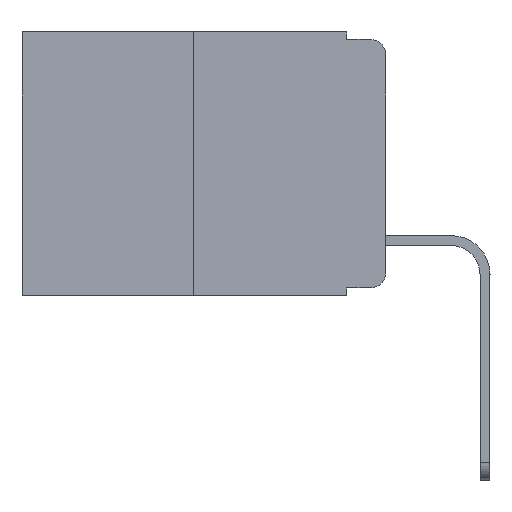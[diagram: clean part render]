
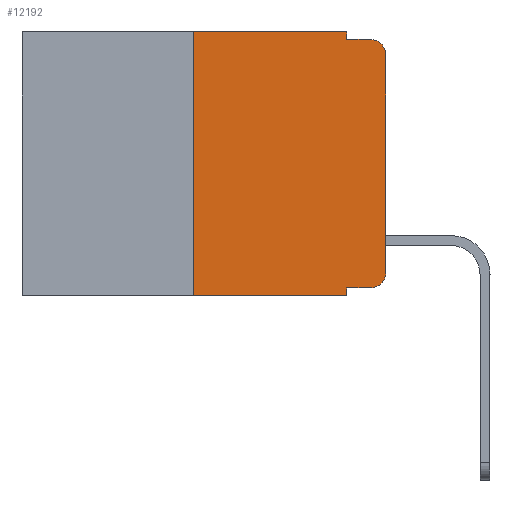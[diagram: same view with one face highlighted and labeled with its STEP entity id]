
A CAD part, left-side view. The second image highlights one B-rep face of the part: STEP entity #12192.
In plain terms, the highlighted planar face has unit normal (-1, 0, 0).
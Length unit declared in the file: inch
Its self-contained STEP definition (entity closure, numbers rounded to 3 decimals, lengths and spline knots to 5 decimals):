
#165 = VECTOR ( 'NONE', #12939, 39.37008 ) ;
#277 = CARTESIAN_POINT ( 'NONE',  ( 0., 0.02, -0.01 ) ) ;
#479 = LINE ( 'NONE', #886, #14516 ) ;
#886 = CARTESIAN_POINT ( 'NONE',  ( 0., 0.473, 0. ) ) ;
#1025 = VERTEX_POINT ( 'NONE', #16205 ) ;
#1231 = VERTEX_POINT ( 'NONE', #7512 ) ;
#1885 = EDGE_LOOP ( 'NONE', ( #11397, #15686, #12711, #11118, #11691, #6294, #12948, #9310, #14647, #5565 ) ) ;
#1897 = EDGE_CURVE ( 'NONE', #12452, #3123, #6984, .T. ) ;
#2125 = VERTEX_POINT ( 'NONE', #277 ) ;
#2444 = CARTESIAN_POINT ( 'NONE',  ( 0., 0.02, -0.313 ) ) ;
#2519 = EDGE_CURVE ( 'NONE', #1231, #14938, #13959, .T. ) ;
#3123 = VERTEX_POINT ( 'NONE', #15446 ) ;
#3140 = DIRECTION ( 'NONE',  ( 0., 0., -1. ) ) ;
#3369 = AXIS2_PLACEMENT_3D ( 'NONE', #10953, #18327, #3140 ) ;
#3494 = VERTEX_POINT ( 'NONE', #17565 ) ;
#3547 = VERTEX_POINT ( 'NONE', #13391 ) ;
#4066 = CARTESIAN_POINT ( 'NONE',  ( 0., 0.051, -0.343 ) ) ;
#4299 = DIRECTION ( 'NONE',  ( 0., -1., 0. ) ) ;
#4918 = FACE_OUTER_BOUND ( 'NONE', #1885, .T. ) ;
#5048 = AXIS2_PLACEMENT_3D ( 'NONE', #2444, #13123, #5357 ) ;
#5357 = DIRECTION ( 'NONE',  ( 0., 0., -1. ) ) ;
#5442 = EDGE_CURVE ( 'NONE', #3123, #2125, #17647, .T. ) ;
#5565 = ORIENTED_EDGE ( 'NONE', *, *, #17591, .T. ) ;
#6294 = ORIENTED_EDGE ( 'NONE', *, *, #13496, .F. ) ;
#6446 = EDGE_CURVE ( 'NONE', #3494, #12452, #479, .T. ) ;
#6984 = LINE ( 'NONE', #12044, #18662 ) ;
#7491 = CARTESIAN_POINT ( 'NONE',  ( 0., 0., -0.03 ) ) ;
#7512 = CARTESIAN_POINT ( 'NONE',  ( 0., 0., -0.313 ) ) ;
#7961 = PLANE ( 'NONE',  #18015 ) ;
#7964 = VERTEX_POINT ( 'NONE', #14975 ) ;
#8744 = VECTOR ( 'NONE', #13066, 39.37008 ) ;
#9214 = CIRCLE ( 'NONE', #3369, 0.02 ) ;
#9310 = ORIENTED_EDGE ( 'NONE', *, *, #12955, .F. ) ;
#9471 = DIRECTION ( 'NONE',  ( 0., -1., 0. ) ) ;
#9487 = EDGE_CURVE ( 'NONE', #7964, #18838, #15745, .T. ) ;
#9700 = CARTESIAN_POINT ( 'NONE',  ( 0., 0.051, -0.333 ) ) ;
#9947 = DIRECTION ( 'NONE',  ( 0., -1., 0. ) ) ;
#10266 = DIRECTION ( 'NONE',  ( 0., 0., -1. ) ) ;
#10455 = VECTOR ( 'NONE', #11415, 39.37008 ) ;
#10953 = CARTESIAN_POINT ( 'NONE',  ( 0., 0.02, -0.03 ) ) ;
#11118 = ORIENTED_EDGE ( 'NONE', *, *, #1897, .F. ) ;
#11397 = ORIENTED_EDGE ( 'NONE', *, *, #2519, .T. ) ;
#11415 = DIRECTION ( 'NONE',  ( 0., -1., 0. ) ) ;
#11676 = CIRCLE ( 'NONE', #5048, 0.02 ) ;
#11691 = ORIENTED_EDGE ( 'NONE', *, *, #6446, .F. ) ;
#12044 = CARTESIAN_POINT ( 'NONE',  ( 0., 0.051, 0. ) ) ;
#12192 = ADVANCED_FACE ( 'NONE', ( #4918 ), #7961, .F. ) ;
#12332 = EDGE_CURVE ( 'NONE', #3547, #1025, #15905, .T. ) ;
#12422 = CARTESIAN_POINT ( 'NONE',  ( 0., 0.473, 0. ) ) ;
#12452 = VERTEX_POINT ( 'NONE', #19185 ) ;
#12711 = ORIENTED_EDGE ( 'NONE', *, *, #5442, .F. ) ;
#12939 = DIRECTION ( 'NONE',  ( 0., 0., 1. ) ) ;
#12948 = ORIENTED_EDGE ( 'NONE', *, *, #9487, .T. ) ;
#12955 = EDGE_CURVE ( 'NONE', #3547, #18838, #13983, .T. ) ;
#13066 = DIRECTION ( 'NONE',  ( 0., 0., -1. ) ) ;
#13123 = DIRECTION ( 'NONE',  ( -1., 0., 0. ) ) ;
#13391 = CARTESIAN_POINT ( 'NONE',  ( 0., 0.051, -0.333 ) ) ;
#13496 = EDGE_CURVE ( 'NONE', #7964, #3494, #15845, .T. ) ;
#13959 = LINE ( 'NONE', #16865, #19175 ) ;
#13983 = LINE ( 'NONE', #15912, #8744 ) ;
#14018 = DIRECTION ( 'NONE',  ( 0., 0., -1. ) ) ;
#14516 = VECTOR ( 'NONE', #9947, 39.37008 ) ;
#14647 = ORIENTED_EDGE ( 'NONE', *, *, #12332, .T. ) ;
#14938 = VERTEX_POINT ( 'NONE', #7491 ) ;
#14975 = CARTESIAN_POINT ( 'NONE',  ( 0., 0.25, -0.343 ) ) ;
#15004 = EDGE_CURVE ( 'NONE', #14938, #2125, #9214, .T. ) ;
#15049 = VECTOR ( 'NONE', #9471, 39.37008 ) ;
#15341 = DIRECTION ( 'NONE',  ( 0., 0., 1. ) ) ;
#15446 = CARTESIAN_POINT ( 'NONE',  ( 0., 0.051, -0.01 ) ) ;
#15686 = ORIENTED_EDGE ( 'NONE', *, *, #15004, .T. ) ;
#15745 = LINE ( 'NONE', #18498, #15049 ) ;
#15845 = LINE ( 'NONE', #16115, #165 ) ;
#15905 = LINE ( 'NONE', #9700, #10455 ) ;
#15912 = CARTESIAN_POINT ( 'NONE',  ( 0., 0.051, 0. ) ) ;
#16115 = CARTESIAN_POINT ( 'NONE',  ( 0., 0.25, 0. ) ) ;
#16205 = CARTESIAN_POINT ( 'NONE',  ( 0., 0.02, -0.333 ) ) ;
#16865 = CARTESIAN_POINT ( 'NONE',  ( 0., 0., 0. ) ) ;
#17565 = CARTESIAN_POINT ( 'NONE',  ( 0., 0.25, 0. ) ) ;
#17591 = EDGE_CURVE ( 'NONE', #1025, #1231, #11676, .T. ) ;
#17647 = LINE ( 'NONE', #19410, #18850 ) ;
#18015 = AXIS2_PLACEMENT_3D ( 'NONE', #12422, #18727, #14018 ) ;
#18327 = DIRECTION ( 'NONE',  ( -1., 0., 0. ) ) ;
#18498 = CARTESIAN_POINT ( 'NONE',  ( 0., 0.473, -0.343 ) ) ;
#18662 = VECTOR ( 'NONE', #10266, 39.37008 ) ;
#18727 = DIRECTION ( 'NONE',  ( 1., 0., 0. ) ) ;
#18838 = VERTEX_POINT ( 'NONE', #4066 ) ;
#18850 = VECTOR ( 'NONE', #4299, 39.37008 ) ;
#19175 = VECTOR ( 'NONE', #15341, 39.37008 ) ;
#19185 = CARTESIAN_POINT ( 'NONE',  ( 0., 0.051, 0. ) ) ;
#19410 = CARTESIAN_POINT ( 'NONE',  ( 0., 0.051, -0.01 ) ) ;
